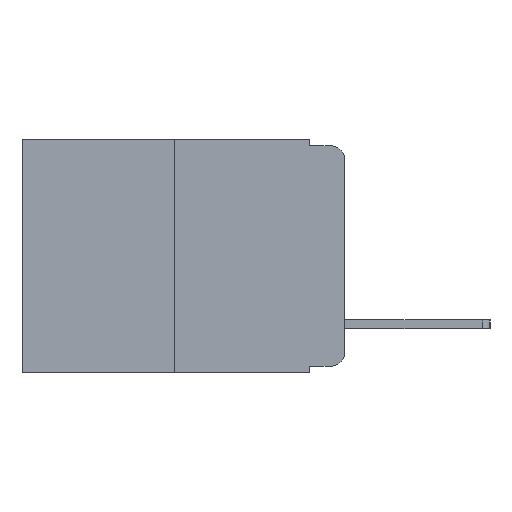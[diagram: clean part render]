
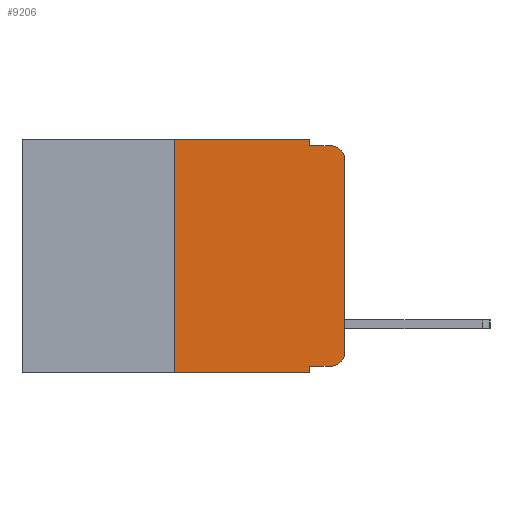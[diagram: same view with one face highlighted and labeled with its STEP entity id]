
A CAD part, left-side view. The second image highlights one B-rep face of the part: STEP entity #9206.
In plain terms, the highlighted planar face has unit normal (-1, 0, 0).
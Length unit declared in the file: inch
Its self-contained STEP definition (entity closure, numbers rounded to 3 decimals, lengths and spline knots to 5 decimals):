
#557 = DIRECTION ( 'NONE',  ( 0., -1., 0. ) ) ;
#1258 = EDGE_CURVE ( 'NONE', #10357, #3329, #15652, .T. ) ;
#1546 = CARTESIAN_POINT ( 'NONE',  ( 0., 0.051, -0.333 ) ) ;
#1726 = LINE ( 'NONE', #18956, #5919 ) ;
#1788 = EDGE_CURVE ( 'NONE', #14738, #10357, #1726, .T. ) ;
#2299 = DIRECTION ( 'NONE',  ( 1., 0., 0. ) ) ;
#2691 = LINE ( 'NONE', #9224, #7350 ) ;
#2815 = VECTOR ( 'NONE', #15811, 39.37008 ) ;
#3098 = VERTEX_POINT ( 'NONE', #13123 ) ;
#3183 = VECTOR ( 'NONE', #3366, 39.37008 ) ;
#3329 = VERTEX_POINT ( 'NONE', #9806 ) ;
#3366 = DIRECTION ( 'NONE',  ( 0., 0., -1. ) ) ;
#3529 = LINE ( 'NONE', #9289, #18358 ) ;
#3726 = VERTEX_POINT ( 'NONE', #15202 ) ;
#4373 = EDGE_CURVE ( 'NONE', #3329, #3726, #8457, .T. ) ;
#4375 = ORIENTED_EDGE ( 'NONE', *, *, #5437, .T. ) ;
#4480 = ORIENTED_EDGE ( 'NONE', *, *, #8516, .T. ) ;
#4767 = ORIENTED_EDGE ( 'NONE', *, *, #1788, .F. ) ;
#4912 = CARTESIAN_POINT ( 'NONE',  ( 0., 0.051, 0. ) ) ;
#5401 = CARTESIAN_POINT ( 'NONE',  ( 0., 0.02, -0.03 ) ) ;
#5437 = EDGE_CURVE ( 'NONE', #3098, #3726, #7008, .T. ) ;
#5730 = ORIENTED_EDGE ( 'NONE', *, *, #1258, .F. ) ;
#5765 = CARTESIAN_POINT ( 'NONE',  ( 0., 0.051, -0.333 ) ) ;
#5919 = VECTOR ( 'NONE', #9528, 39.37008 ) ;
#6000 = CARTESIAN_POINT ( 'NONE',  ( 0., 0.02, -0.333 ) ) ;
#6401 = VERTEX_POINT ( 'NONE', #17712 ) ;
#6976 = DIRECTION ( 'NONE',  ( 0., 0., -1. ) ) ;
#6989 = PLANE ( 'NONE',  #10512 ) ;
#7008 = CIRCLE ( 'NONE', #14875, 0.02 ) ;
#7090 = VERTEX_POINT ( 'NONE', #19300 ) ;
#7191 = VECTOR ( 'NONE', #11208, 39.37008 ) ;
#7350 = VECTOR ( 'NONE', #16483, 39.37008 ) ;
#7669 = LINE ( 'NONE', #18357, #7191 ) ;
#7732 = DIRECTION ( 'NONE',  ( 0., 0., -1. ) ) ;
#8457 = LINE ( 'NONE', #12155, #15786 ) ;
#8516 = EDGE_CURVE ( 'NONE', #7090, #3098, #14854, .T. ) ;
#8520 = CARTESIAN_POINT ( 'NONE',  ( 0., 0., 0. ) ) ;
#8927 = DIRECTION ( 'NONE',  ( -1., 0., 0. ) ) ;
#9206 = ADVANCED_FACE ( 'NONE', ( #18162 ), #6989, .F. ) ;
#9224 = CARTESIAN_POINT ( 'NONE',  ( 0., 0.473, -0.343 ) ) ;
#9289 = CARTESIAN_POINT ( 'NONE',  ( 0., 0.051, 0. ) ) ;
#9478 = CIRCLE ( 'NONE', #16968, 0.02 ) ;
#9528 = DIRECTION ( 'NONE',  ( 0., -1., 0. ) ) ;
#9806 = CARTESIAN_POINT ( 'NONE',  ( 0., 0.051, -0.01 ) ) ;
#10357 = VERTEX_POINT ( 'NONE', #15883 ) ;
#10494 = ORIENTED_EDGE ( 'NONE', *, *, #4373, .F. ) ;
#10512 = AXIS2_PLACEMENT_3D ( 'NONE', #18590, #2299, #12963 ) ;
#11208 = DIRECTION ( 'NONE',  ( 0., 0., 1. ) ) ;
#11211 = VERTEX_POINT ( 'NONE', #5765 ) ;
#11237 = VECTOR ( 'NONE', #16573, 39.37008 ) ;
#11859 = EDGE_CURVE ( 'NONE', #16373, #7090, #9478, .T. ) ;
#12155 = CARTESIAN_POINT ( 'NONE',  ( 0., 0.051, -0.01 ) ) ;
#12638 = EDGE_CURVE ( 'NONE', #17729, #6401, #2691, .T. ) ;
#12658 = ORIENTED_EDGE ( 'NONE', *, *, #11859, .T. ) ;
#12963 = DIRECTION ( 'NONE',  ( 0., 0., -1. ) ) ;
#13031 = EDGE_LOOP ( 'NONE', ( #4480, #4375, #10494, #5730, #4767, #13316, #16461, #17639, #15275, #12658 ) ) ;
#13123 = CARTESIAN_POINT ( 'NONE',  ( 0., 0., -0.03 ) ) ;
#13316 = ORIENTED_EDGE ( 'NONE', *, *, #16699, .F. ) ;
#13800 = EDGE_CURVE ( 'NONE', #11211, #16373, #15119, .T. ) ;
#14738 = VERTEX_POINT ( 'NONE', #14982 ) ;
#14786 = EDGE_CURVE ( 'NONE', #11211, #6401, #3529, .T. ) ;
#14854 = LINE ( 'NONE', #8520, #2815 ) ;
#14875 = AXIS2_PLACEMENT_3D ( 'NONE', #5401, #15780, #6976 ) ;
#14982 = CARTESIAN_POINT ( 'NONE',  ( 0., 0.25, 0. ) ) ;
#15119 = LINE ( 'NONE', #1546, #11237 ) ;
#15202 = CARTESIAN_POINT ( 'NONE',  ( 0., 0.02, -0.01 ) ) ;
#15275 = ORIENTED_EDGE ( 'NONE', *, *, #13800, .T. ) ;
#15652 = LINE ( 'NONE', #4912, #3183 ) ;
#15780 = DIRECTION ( 'NONE',  ( -1., 0., 0. ) ) ;
#15786 = VECTOR ( 'NONE', #557, 39.37008 ) ;
#15811 = DIRECTION ( 'NONE',  ( 0., 0., 1. ) ) ;
#15883 = CARTESIAN_POINT ( 'NONE',  ( 0., 0.051, 0. ) ) ;
#16373 = VERTEX_POINT ( 'NONE', #6000 ) ;
#16461 = ORIENTED_EDGE ( 'NONE', *, *, #12638, .T. ) ;
#16483 = DIRECTION ( 'NONE',  ( 0., -1., 0. ) ) ;
#16573 = DIRECTION ( 'NONE',  ( 0., -1., 0. ) ) ;
#16699 = EDGE_CURVE ( 'NONE', #17729, #14738, #7669, .T. ) ;
#16968 = AXIS2_PLACEMENT_3D ( 'NONE', #17606, #8927, #18996 ) ;
#17606 = CARTESIAN_POINT ( 'NONE',  ( 0., 0.02, -0.313 ) ) ;
#17639 = ORIENTED_EDGE ( 'NONE', *, *, #14786, .F. ) ;
#17712 = CARTESIAN_POINT ( 'NONE',  ( 0., 0.051, -0.343 ) ) ;
#17729 = VERTEX_POINT ( 'NONE', #18211 ) ;
#18162 = FACE_OUTER_BOUND ( 'NONE', #13031, .T. ) ;
#18211 = CARTESIAN_POINT ( 'NONE',  ( 0., 0.25, -0.343 ) ) ;
#18357 = CARTESIAN_POINT ( 'NONE',  ( 0., 0.25, 0. ) ) ;
#18358 = VECTOR ( 'NONE', #7732, 39.37008 ) ;
#18590 = CARTESIAN_POINT ( 'NONE',  ( 0., 0.473, 0. ) ) ;
#18956 = CARTESIAN_POINT ( 'NONE',  ( 0., 0.473, 0. ) ) ;
#18996 = DIRECTION ( 'NONE',  ( 0., 0., -1. ) ) ;
#19300 = CARTESIAN_POINT ( 'NONE',  ( 0., 0., -0.313 ) ) ;
